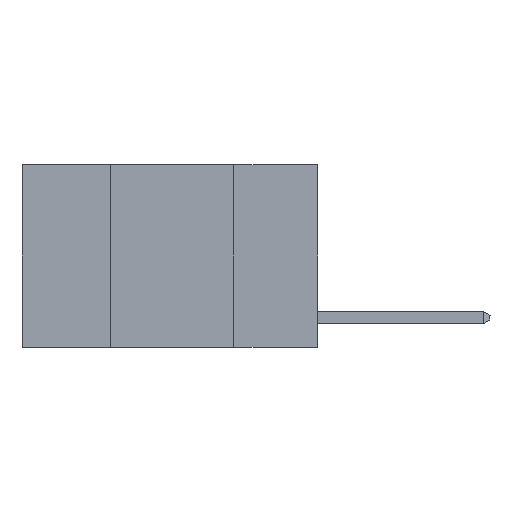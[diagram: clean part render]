
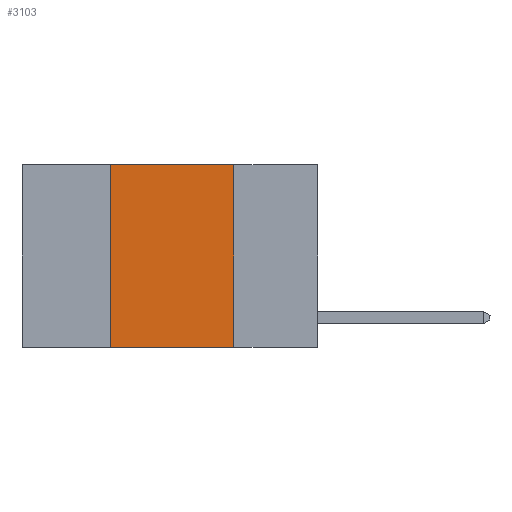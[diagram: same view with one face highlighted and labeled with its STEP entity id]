
A CAD part, left-side view. The second image highlights one B-rep face of the part: STEP entity #3103.
In plain terms, the highlighted planar face has unit normal (-1, 0, 0).
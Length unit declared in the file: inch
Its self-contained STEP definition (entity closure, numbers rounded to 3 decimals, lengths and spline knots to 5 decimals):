
#49 = ORIENTED_EDGE ( 'NONE', *, *, #7003, .F. ) ;
#177 = CARTESIAN_POINT ( 'NONE',  ( 0., 0.42, 0. ) ) ;
#784 = LINE ( 'NONE', #5899, #10622 ) ;
#1191 = DIRECTION ( 'NONE',  ( 0., 0., 1. ) ) ;
#1430 = PLANE ( 'NONE',  #12140 ) ;
#2866 = CARTESIAN_POINT ( 'NONE',  ( 0., 0.17, -0.37 ) ) ;
#2944 = LINE ( 'NONE', #11501, #10177 ) ;
#3103 = ADVANCED_FACE ( 'NONE', ( #9556 ), #1430, .F. ) ;
#3461 = CARTESIAN_POINT ( 'NONE',  ( 0., 0.6, 0. ) ) ;
#3895 = DIRECTION ( 'NONE',  ( 0., 0., -1. ) ) ;
#3932 = ORIENTED_EDGE ( 'NONE', *, *, #7645, .F. ) ;
#4249 = VECTOR ( 'NONE', #8923, 39.37008 ) ;
#4514 = DIRECTION ( 'NONE',  ( 0., 0., -1. ) ) ;
#5762 = CARTESIAN_POINT ( 'NONE',  ( 0., 0.6, 0. ) ) ;
#5842 = EDGE_LOOP ( 'NONE', ( #49, #3932, #6884, #8333 ) ) ;
#5899 = CARTESIAN_POINT ( 'NONE',  ( 0., 0.17, 0. ) ) ;
#5980 = VERTEX_POINT ( 'NONE', #11619 ) ;
#6007 = LINE ( 'NONE', #5762, #8163 ) ;
#6884 = ORIENTED_EDGE ( 'NONE', *, *, #7283, .F. ) ;
#7003 = EDGE_CURVE ( 'NONE', #5980, #7041, #784, .T. ) ;
#7041 = VERTEX_POINT ( 'NONE', #2866 ) ;
#7283 = EDGE_CURVE ( 'NONE', #8115, #10187, #2944, .T. ) ;
#7645 = EDGE_CURVE ( 'NONE', #10187, #5980, #6007, .T. ) ;
#7999 = EDGE_CURVE ( 'NONE', #8115, #7041, #11510, .T. ) ;
#8064 = CARTESIAN_POINT ( 'NONE',  ( 0., 0.6, -0.37 ) ) ;
#8115 = VERTEX_POINT ( 'NONE', #9902 ) ;
#8163 = VECTOR ( 'NONE', #8529, 39.37008 ) ;
#8333 = ORIENTED_EDGE ( 'NONE', *, *, #7999, .T. ) ;
#8529 = DIRECTION ( 'NONE',  ( 0., -1., 0. ) ) ;
#8923 = DIRECTION ( 'NONE',  ( 0., -1., 0. ) ) ;
#9556 = FACE_OUTER_BOUND ( 'NONE', #5842, .T. ) ;
#9902 = CARTESIAN_POINT ( 'NONE',  ( 0., 0.42, -0.37 ) ) ;
#10027 = DIRECTION ( 'NONE',  ( 1., 0., 0. ) ) ;
#10177 = VECTOR ( 'NONE', #1191, 39.37008 ) ;
#10187 = VERTEX_POINT ( 'NONE', #177 ) ;
#10622 = VECTOR ( 'NONE', #3895, 39.37008 ) ;
#11501 = CARTESIAN_POINT ( 'NONE',  ( 0., 0.42, 0. ) ) ;
#11510 = LINE ( 'NONE', #8064, #4249 ) ;
#11619 = CARTESIAN_POINT ( 'NONE',  ( 0., 0.17, 0. ) ) ;
#12140 = AXIS2_PLACEMENT_3D ( 'NONE', #3461, #10027, #4514 ) ;
